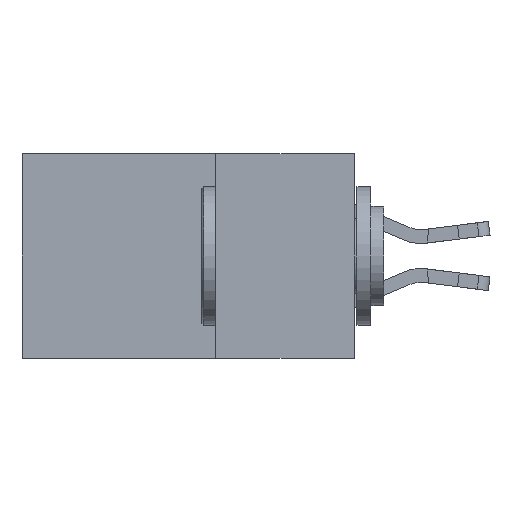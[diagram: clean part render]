
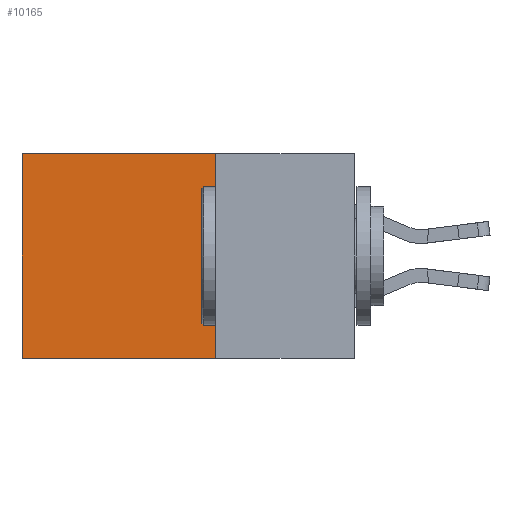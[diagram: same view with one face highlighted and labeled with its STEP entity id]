
A CAD part, left-side view. The second image highlights one B-rep face of the part: STEP entity #10165.
In plain terms, the highlighted planar face has unit normal (-1, 0, 0).
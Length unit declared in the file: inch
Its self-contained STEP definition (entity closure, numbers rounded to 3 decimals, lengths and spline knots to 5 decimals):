
#371 = CARTESIAN_POINT ( 'NONE',  ( 0.298, 0.25, -0.37 ) ) ;
#681 = CARTESIAN_POINT ( 'NONE',  ( 0.298, 0.25, 0. ) ) ;
#3116 = DIRECTION ( 'NONE',  ( 0., 0., -1. ) ) ;
#3852 = LINE ( 'NONE', #24771, #24906 ) ;
#3928 = CARTESIAN_POINT ( 'NONE',  ( 0.298, 0.25, -0.37 ) ) ;
#4552 = CARTESIAN_POINT ( 'NONE',  ( 0.298, 0.6, 0. ) ) ;
#5255 = VECTOR ( 'NONE', #18900, 39.37008 ) ;
#5738 = CARTESIAN_POINT ( 'NONE',  ( 0.298, 0.6, -0.37 ) ) ;
#5816 = LINE ( 'NONE', #17558, #11261 ) ;
#6618 = LINE ( 'NONE', #371, #5255 ) ;
#6931 = VERTEX_POINT ( 'NONE', #17898 ) ;
#7620 = VERTEX_POINT ( 'NONE', #5738 ) ;
#7629 = LINE ( 'NONE', #4552, #22473 ) ;
#9198 = EDGE_CURVE ( 'NONE', #10327, #7620, #6618, .T. ) ;
#9739 = PLANE ( 'NONE',  #11711 ) ;
#10165 = ADVANCED_FACE ( 'NONE', ( #24252 ), #9739, .F. ) ;
#10327 = VERTEX_POINT ( 'NONE', #3928 ) ;
#10770 = DIRECTION ( 'NONE',  ( 0., 1., 0. ) ) ;
#11085 = ORIENTED_EDGE ( 'NONE', *, *, #14087, .T. ) ;
#11261 = VECTOR ( 'NONE', #3116, 39.37008 ) ;
#11356 = ORIENTED_EDGE ( 'NONE', *, *, #9198, .F. ) ;
#11559 = EDGE_LOOP ( 'NONE', ( #11085, #11356, #20034, #15711 ) ) ;
#11711 = AXIS2_PLACEMENT_3D ( 'NONE', #23835, #25823, #13811 ) ;
#13811 = DIRECTION ( 'NONE',  ( 0., 0., -1. ) ) ;
#14087 = EDGE_CURVE ( 'NONE', #6931, #7620, #7629, .T. ) ;
#14808 = DIRECTION ( 'NONE',  ( 0., 0., -1. ) ) ;
#15300 = EDGE_CURVE ( 'NONE', #22639, #6931, #3852, .T. ) ;
#15711 = ORIENTED_EDGE ( 'NONE', *, *, #15300, .T. ) ;
#17558 = CARTESIAN_POINT ( 'NONE',  ( 0.298, 0.25, 0. ) ) ;
#17898 = CARTESIAN_POINT ( 'NONE',  ( 0.298, 0.6, 0. ) ) ;
#18900 = DIRECTION ( 'NONE',  ( 0., 1., 0. ) ) ;
#20034 = ORIENTED_EDGE ( 'NONE', *, *, #24694, .F. ) ;
#22473 = VECTOR ( 'NONE', #14808, 39.37008 ) ;
#22639 = VERTEX_POINT ( 'NONE', #681 ) ;
#23835 = CARTESIAN_POINT ( 'NONE',  ( 0.298, 0.25, 0. ) ) ;
#24252 = FACE_OUTER_BOUND ( 'NONE', #11559, .T. ) ;
#24694 = EDGE_CURVE ( 'NONE', #22639, #10327, #5816, .T. ) ;
#24771 = CARTESIAN_POINT ( 'NONE',  ( 0.298, 0.25, 0. ) ) ;
#24906 = VECTOR ( 'NONE', #10770, 39.37008 ) ;
#25823 = DIRECTION ( 'NONE',  ( 1., 0., 0. ) ) ;
